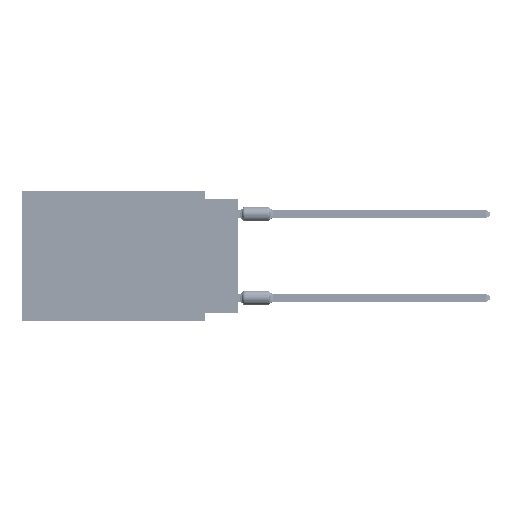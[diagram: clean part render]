
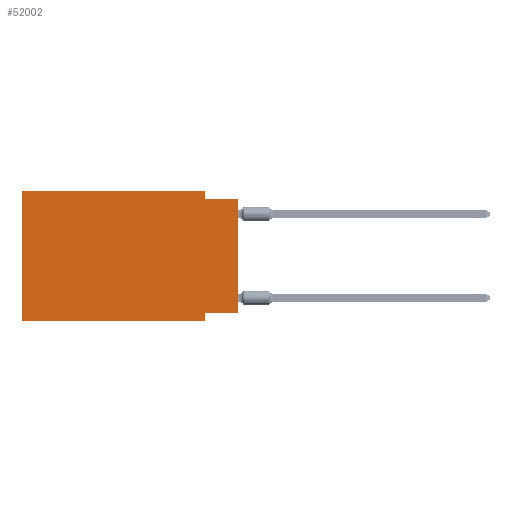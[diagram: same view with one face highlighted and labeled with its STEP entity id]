
A CAD part, left-side view. The second image highlights one B-rep face of the part: STEP entity #52002.
In plain terms, the highlighted planar face has unit normal (-1, 0, 0).
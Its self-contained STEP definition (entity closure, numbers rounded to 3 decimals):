
#379 = CARTESIAN_POINT ( 'NONE',  ( 0., 0., -9.271 ) ) ;
#1017 = EDGE_CURVE ( 'NONE', #29327, #57018, #37243, .T. ) ;
#1985 = DIRECTION ( 'NONE',  ( 0., 0., 1. ) ) ;
#2238 = VECTOR ( 'NONE', #22434, 1000. ) ;
#3880 = CARTESIAN_POINT ( 'NONE',  ( 0., 0., -0.635 ) ) ;
#5239 = DIRECTION ( 'NONE',  ( 0., -1., 0. ) ) ;
#5475 = DIRECTION ( 'NONE',  ( 0., 0., -1. ) ) ;
#6140 = AXIS2_PLACEMENT_3D ( 'NONE', #67552, #30172, #35752 ) ;
#7244 = CARTESIAN_POINT ( 'NONE',  ( 0., 2.54, -9.271 ) ) ;
#8872 = FACE_OUTER_BOUND ( 'NONE', #27768, .T. ) ;
#9004 = VERTEX_POINT ( 'NONE', #7244 ) ;
#10548 = CARTESIAN_POINT ( 'NONE',  ( 0., 2.54, -0.635 ) ) ;
#10762 = ORIENTED_EDGE ( 'NONE', *, *, #1017, .F. ) ;
#11222 = VECTOR ( 'NONE', #1985, 1000. ) ;
#12388 = ORIENTED_EDGE ( 'NONE', *, *, #33150, .F. ) ;
#16075 = EDGE_CURVE ( 'NONE', #54673, #41086, #26534, .T. ) ;
#16692 = EDGE_CURVE ( 'NONE', #54673, #54424, #17688, .T. ) ;
#17116 = CARTESIAN_POINT ( 'NONE',  ( 0., 0., 0. ) ) ;
#17188 = LINE ( 'NONE', #23453, #2238 ) ;
#17688 = LINE ( 'NONE', #60291, #11222 ) ;
#22434 = DIRECTION ( 'NONE',  ( 0., 0., -1. ) ) ;
#23453 = CARTESIAN_POINT ( 'NONE',  ( 0., 2.54, -9.906 ) ) ;
#23698 = CARTESIAN_POINT ( 'NONE',  ( 0., 16.383, 0. ) ) ;
#26534 = LINE ( 'NONE', #57629, #57972 ) ;
#27768 = EDGE_LOOP ( 'NONE', ( #64839, #36982, #10762, #50118, #36524, #53720, #12388, #57087 ) ) ;
#29327 = VERTEX_POINT ( 'NONE', #56010 ) ;
#30172 = DIRECTION ( 'NONE',  ( 1., 0., 0. ) ) ;
#30425 = LINE ( 'NONE', #3880, #51493 ) ;
#32011 = CARTESIAN_POINT ( 'NONE',  ( 0., 2.54, 0. ) ) ;
#32401 = EDGE_CURVE ( 'NONE', #54424, #29327, #46647, .T. ) ;
#33150 = EDGE_CURVE ( 'NONE', #9004, #41086, #17188, .T. ) ;
#33503 = LINE ( 'NONE', #17116, #35023 ) ;
#34189 = DIRECTION ( 'NONE',  ( 0., 0., 1. ) ) ;
#34467 = EDGE_CURVE ( 'NONE', #57018, #60366, #30425, .T. ) ;
#34506 = DIRECTION ( 'NONE',  ( 0., -1., 0. ) ) ;
#35023 = VECTOR ( 'NONE', #34189, 1000. ) ;
#35752 = DIRECTION ( 'NONE',  ( 0., 0., -1. ) ) ;
#36191 = CARTESIAN_POINT ( 'NONE',  ( 0., 0., -9.271 ) ) ;
#36524 = ORIENTED_EDGE ( 'NONE', *, *, #16692, .F. ) ;
#36982 = ORIENTED_EDGE ( 'NONE', *, *, #34467, .F. ) ;
#37243 = LINE ( 'NONE', #32011, #54011 ) ;
#38823 = EDGE_CURVE ( 'NONE', #52752, #9004, #68825, .T. ) ;
#40758 = CARTESIAN_POINT ( 'NONE',  ( 0., 16.383, -9.906 ) ) ;
#40896 = DIRECTION ( 'NONE',  ( 0., -1., 0. ) ) ;
#41086 = VERTEX_POINT ( 'NONE', #61535 ) ;
#45129 = CARTESIAN_POINT ( 'NONE',  ( 0., 0., -0.635 ) ) ;
#46647 = LINE ( 'NONE', #23698, #52176 ) ;
#50118 = ORIENTED_EDGE ( 'NONE', *, *, #32401, .F. ) ;
#50810 = CARTESIAN_POINT ( 'NONE',  ( 0., 16.383, 0. ) ) ;
#51054 = EDGE_CURVE ( 'NONE', #52752, #60366, #33503, .T. ) ;
#51493 = VECTOR ( 'NONE', #40896, 1000. ) ;
#52002 = ADVANCED_FACE ( 'NONE', ( #8872 ), #61260, .F. ) ;
#52176 = VECTOR ( 'NONE', #34506, 1000. ) ;
#52752 = VERTEX_POINT ( 'NONE', #36191 ) ;
#53720 = ORIENTED_EDGE ( 'NONE', *, *, #16075, .T. ) ;
#54011 = VECTOR ( 'NONE', #5475, 1000. ) ;
#54424 = VERTEX_POINT ( 'NONE', #50810 ) ;
#54673 = VERTEX_POINT ( 'NONE', #40758 ) ;
#56010 = CARTESIAN_POINT ( 'NONE',  ( 0., 2.54, 0. ) ) ;
#57018 = VERTEX_POINT ( 'NONE', #10548 ) ;
#57087 = ORIENTED_EDGE ( 'NONE', *, *, #38823, .F. ) ;
#57629 = CARTESIAN_POINT ( 'NONE',  ( 0., 16.383, -9.906 ) ) ;
#57972 = VECTOR ( 'NONE', #5239, 1000. ) ;
#60291 = CARTESIAN_POINT ( 'NONE',  ( 0., 16.383, 0. ) ) ;
#60366 = VERTEX_POINT ( 'NONE', #45129 ) ;
#61260 = PLANE ( 'NONE',  #6140 ) ;
#61535 = CARTESIAN_POINT ( 'NONE',  ( 0., 2.54, -9.906 ) ) ;
#64276 = DIRECTION ( 'NONE',  ( 0., 1., 0. ) ) ;
#64839 = ORIENTED_EDGE ( 'NONE', *, *, #51054, .T. ) ;
#66172 = VECTOR ( 'NONE', #64276, 1000. ) ;
#67552 = CARTESIAN_POINT ( 'NONE',  ( 0., 16.383, 0. ) ) ;
#68825 = LINE ( 'NONE', #379, #66172 ) ;
